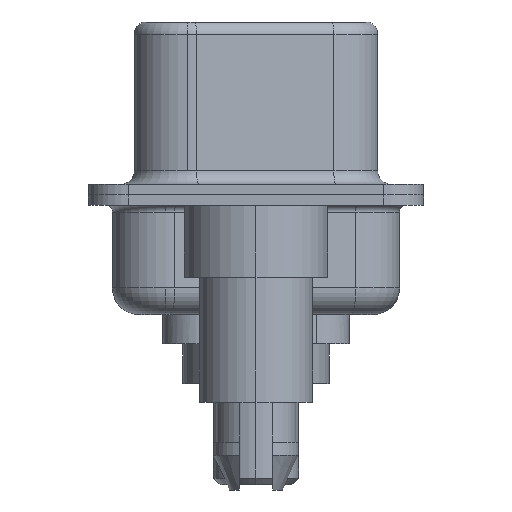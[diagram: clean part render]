
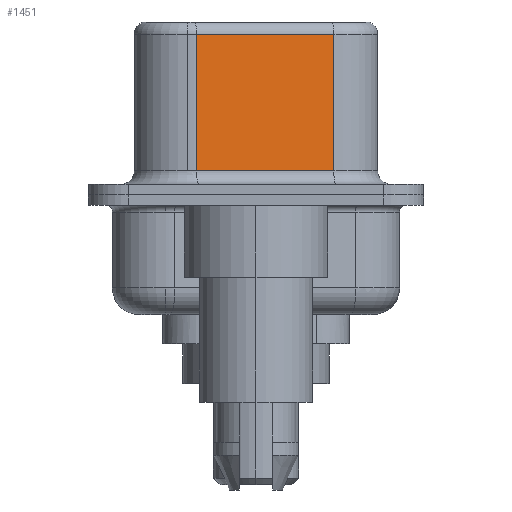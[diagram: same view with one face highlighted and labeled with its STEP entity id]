
A CAD part, left-side view. The second image highlights one B-rep face of the part: STEP entity #1451.
In plain terms, the highlighted planar face has unit normal (-0.985, -0.174, 0).
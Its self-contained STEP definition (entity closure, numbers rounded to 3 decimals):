
#69 = EDGE_CURVE ( 'NONE', #3221, #12562, #6916, .T. ) ;
#158 = LINE ( 'NONE', #4341, #12035 ) ;
#341 = CARTESIAN_POINT ( 'NONE',  ( 3.655, 2.233, 6.52 ) ) ;
#921 = AXIS2_PLACEMENT_3D ( 'NONE', #4733, #4995, #14404 ) ;
#1451 = ADVANCED_FACE ( 'NONE', ( #4897 ), #13803, .F. ) ;
#1911 = DIRECTION ( 'NONE',  ( 0., 0., -1. ) ) ;
#2513 = DIRECTION ( 'NONE',  ( 0.174, -0.985, 0. ) ) ;
#2712 = VERTEX_POINT ( 'NONE', #11781 ) ;
#2957 = DIRECTION ( 'NONE',  ( -0.174, 0.985, 0. ) ) ;
#2997 = CARTESIAN_POINT ( 'NONE',  ( 4.565, -2.927, 6.02 ) ) ;
#3221 = VERTEX_POINT ( 'NONE', #14072 ) ;
#3504 = VECTOR ( 'NONE', #2957, 1000. ) ;
#3897 = ORIENTED_EDGE ( 'NONE', *, *, #13504, .T. ) ;
#4341 = CARTESIAN_POINT ( 'NONE',  ( 4.565, -2.927, 6.52 ) ) ;
#4492 = VECTOR ( 'NONE', #2513, 1000. ) ;
#4733 = CARTESIAN_POINT ( 'NONE',  ( 4.565, -2.927, 6.52 ) ) ;
#4897 = FACE_OUTER_BOUND ( 'NONE', #11458, .T. ) ;
#4995 = DIRECTION ( 'NONE',  ( 0.985, 0.174, 0. ) ) ;
#5172 = EDGE_CURVE ( 'NONE', #3221, #2712, #158, .T. ) ;
#5517 = CARTESIAN_POINT ( 'NONE',  ( 3.655, 2.233, 0.9 ) ) ;
#6745 = DIRECTION ( 'NONE',  ( 0., 0., -1. ) ) ;
#6916 = LINE ( 'NONE', #2997, #3504 ) ;
#7583 = CARTESIAN_POINT ( 'NONE',  ( 4.565, -2.927, 0.9 ) ) ;
#7817 = LINE ( 'NONE', #7583, #4492 ) ;
#10073 = CARTESIAN_POINT ( 'NONE',  ( 3.655, 2.233, 6.02 ) ) ;
#10167 = LINE ( 'NONE', #341, #13545 ) ;
#11458 = EDGE_LOOP ( 'NONE', ( #14165, #11820, #14884, #3897 ) ) ;
#11781 = CARTESIAN_POINT ( 'NONE',  ( 4.565, -2.927, 0.9 ) ) ;
#11820 = ORIENTED_EDGE ( 'NONE', *, *, #69, .T. ) ;
#12035 = VECTOR ( 'NONE', #1911, 1000. ) ;
#12562 = VERTEX_POINT ( 'NONE', #10073 ) ;
#12770 = EDGE_CURVE ( 'NONE', #12562, #14963, #10167, .T. ) ;
#13504 = EDGE_CURVE ( 'NONE', #14963, #2712, #7817, .T. ) ;
#13545 = VECTOR ( 'NONE', #6745, 1000. ) ;
#13803 = PLANE ( 'NONE',  #921 ) ;
#14072 = CARTESIAN_POINT ( 'NONE',  ( 4.565, -2.927, 6.02 ) ) ;
#14165 = ORIENTED_EDGE ( 'NONE', *, *, #5172, .F. ) ;
#14404 = DIRECTION ( 'NONE',  ( -0.174, 0.985, 0. ) ) ;
#14884 = ORIENTED_EDGE ( 'NONE', *, *, #12770, .T. ) ;
#14963 = VERTEX_POINT ( 'NONE', #5517 ) ;
